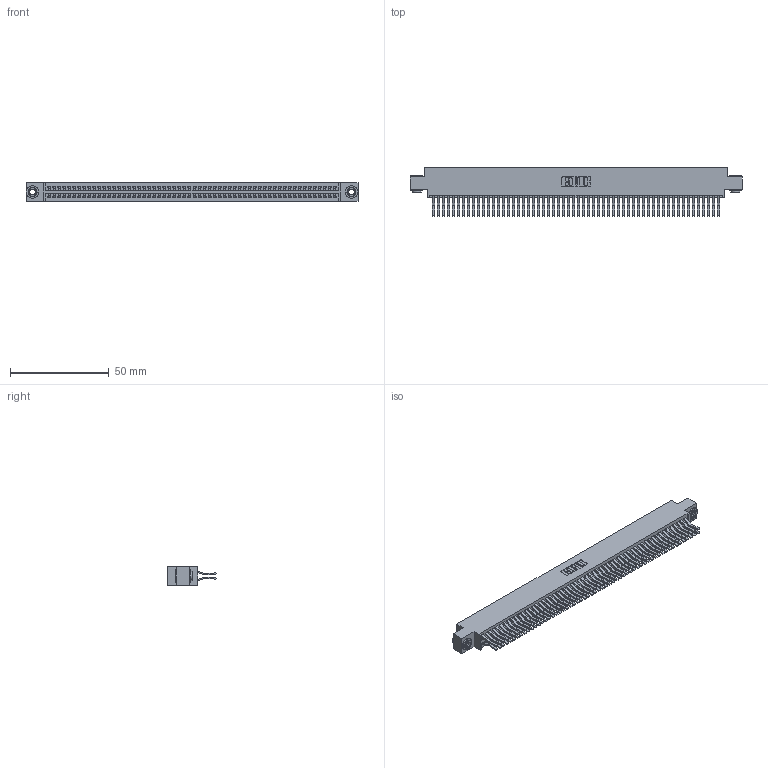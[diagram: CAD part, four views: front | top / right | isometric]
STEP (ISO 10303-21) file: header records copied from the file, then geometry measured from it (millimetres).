
FILE_DESCRIPTION (( 'STEP AP203' ), '1' );
FILE_NAME ('395-116-560-803.STEP', '2018-12-02T04:14:16', ( '' ), ( '' ), 'SwSTEP 2.0', 'SolidWorks 2016', '' );
FILE_SCHEMA (( 'CONFIG_CONTROL_DESIGN' ));
Length unit declared in the file: inch
Products named in the file (4): 345-292-001_560 Tail; 395-116-560-803; 345-250-002_345-250-002-102; 345 Part_0.170 Offset - 0.156 Dia-TH
Assembly tree (119 placements, depth 2):
  395-116-560-803
    345 Part_0.170 Offset - 0.156 Dia-TH
    345-292-001_560 Tail  x116
    345-250-002_345-250-002-102  x2
Bounding box: 168.53 x 24.45 x 9.4 mm (x, y, z)
Volume: 17185.9 mm3; surface area: 28017.5 mm2
Topology: 119 solids, 119 shells, 6200 faces, 18409 edges, 12114 vertices
Faces by surface type: plane 3922, cylinder 2270, cone 8
Entity records: 44224 total; most frequent: CARTESIAN_POINT 7375, ORIENTED_EDGE 7302, DIRECTION 6517, EDGE_CURVE 3651, VECTOR 3259, LINE 3259, VERTEX_POINT 2430, AXIS2_PLACEMENT_3D 1629
